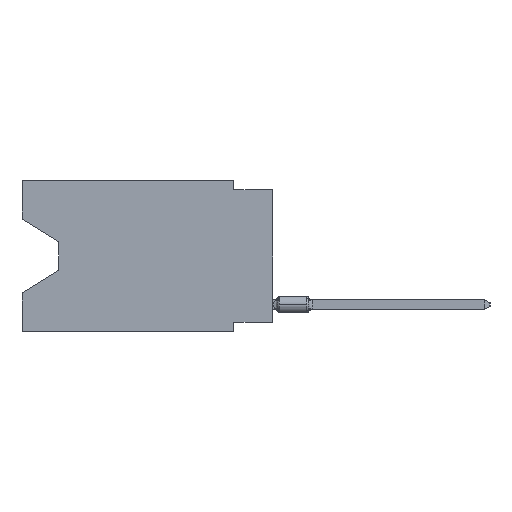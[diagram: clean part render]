
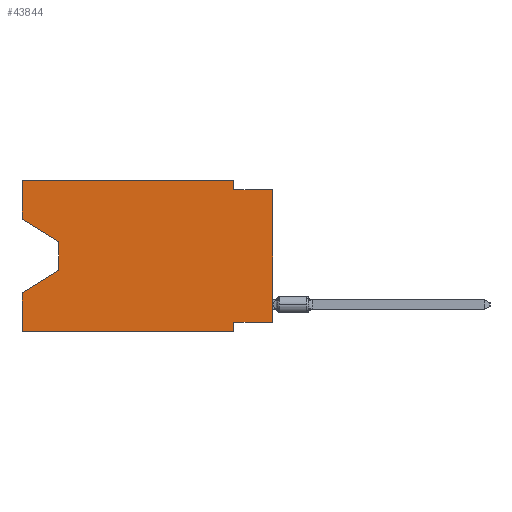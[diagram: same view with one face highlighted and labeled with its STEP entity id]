
A CAD part, left-side view. The second image highlights one B-rep face of the part: STEP entity #43844.
In plain terms, the highlighted planar face has unit normal (-1, 0, 0).
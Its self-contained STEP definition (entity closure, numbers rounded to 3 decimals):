
#414 = LINE ( 'NONE', #41570, #20979 ) ;
#594 = LINE ( 'NONE', #4334, #33342 ) ;
#1534 = DIRECTION ( 'NONE',  ( 0., 0., -1. ) ) ;
#2400 = ORIENTED_EDGE ( 'NONE', *, *, #45570, .F. ) ;
#2598 = DIRECTION ( 'NONE',  ( 1., 0., 0. ) ) ;
#3340 = CARTESIAN_POINT ( 'NONE',  ( 0., 2.54, -9.906 ) ) ;
#4219 = EDGE_CURVE ( 'NONE', #40050, #27519, #4871, .T. ) ;
#4334 = CARTESIAN_POINT ( 'NONE',  ( 0., 13.97, -5.893 ) ) ;
#4600 = DIRECTION ( 'NONE',  ( 0., 1., 0. ) ) ;
#4824 = LINE ( 'NONE', #29526, #19362 ) ;
#4871 = LINE ( 'NONE', #29850, #43317 ) ;
#5742 = CARTESIAN_POINT ( 'NONE',  ( 0., 2.54, 0. ) ) ;
#6834 = AXIS2_PLACEMENT_3D ( 'NONE', #39268, #2598, #22293 ) ;
#7279 = VECTOR ( 'NONE', #7648, 1000. ) ;
#7379 = LINE ( 'NONE', #43779, #7279 ) ;
#7648 = DIRECTION ( 'NONE',  ( 0., 0., 1. ) ) ;
#7811 = CARTESIAN_POINT ( 'NONE',  ( 0., 16.383, -7.36 ) ) ;
#8549 = DIRECTION ( 'NONE',  ( 0., -1., 0. ) ) ;
#8772 = ORIENTED_EDGE ( 'NONE', *, *, #42619, .F. ) ;
#8884 = EDGE_CURVE ( 'NONE', #28193, #33493, #33404, .T. ) ;
#9623 = LINE ( 'NONE', #21852, #44292 ) ;
#9801 = VERTEX_POINT ( 'NONE', #40774 ) ;
#9888 = EDGE_CURVE ( 'NONE', #28742, #27519, #44262, .T. ) ;
#12550 = LINE ( 'NONE', #24804, #28298 ) ;
#12706 = CARTESIAN_POINT ( 'NONE',  ( 0., 2.54, -9.906 ) ) ;
#13138 = CARTESIAN_POINT ( 'NONE',  ( 0., 2.54, -0.635 ) ) ;
#13321 = ORIENTED_EDGE ( 'NONE', *, *, #9888, .F. ) ;
#15783 = CARTESIAN_POINT ( 'NONE',  ( 0., 16.383, -2.546 ) ) ;
#15956 = VERTEX_POINT ( 'NONE', #13138 ) ;
#16697 = CARTESIAN_POINT ( 'NONE',  ( 0., 16.383, 0. ) ) ;
#19323 = CARTESIAN_POINT ( 'NONE',  ( 0., 16.383, -9.906 ) ) ;
#19362 = VECTOR ( 'NONE', #8549, 1000. ) ;
#19572 = DIRECTION ( 'NONE',  ( 0., 0., -1. ) ) ;
#20979 = VECTOR ( 'NONE', #41314, 1000. ) ;
#21483 = VERTEX_POINT ( 'NONE', #49431 ) ;
#21852 = CARTESIAN_POINT ( 'NONE',  ( 0., 16.383, 0. ) ) ;
#22277 = LINE ( 'NONE', #26261, #51580 ) ;
#22293 = DIRECTION ( 'NONE',  ( 0., 0., -1. ) ) ;
#22459 = LINE ( 'NONE', #47402, #42807 ) ;
#23095 = FACE_OUTER_BOUND ( 'NONE', #48795, .T. ) ;
#23185 = EDGE_CURVE ( 'NONE', #33493, #15956, #22277, .T. ) ;
#24553 = VECTOR ( 'NONE', #27745, 1000. ) ;
#24804 = CARTESIAN_POINT ( 'NONE',  ( 0., 0., -9.271 ) ) ;
#26261 = CARTESIAN_POINT ( 'NONE',  ( 0., 2.54, 0. ) ) ;
#26876 = EDGE_CURVE ( 'NONE', #30911, #21483, #22459, .T. ) ;
#27298 = ORIENTED_EDGE ( 'NONE', *, *, #35613, .F. ) ;
#27519 = VERTEX_POINT ( 'NONE', #12706 ) ;
#27745 = DIRECTION ( 'NONE',  ( 0., -0.855, -0.519 ) ) ;
#28193 = VERTEX_POINT ( 'NONE', #47946 ) ;
#28298 = VECTOR ( 'NONE', #4600, 1000. ) ;
#28742 = VERTEX_POINT ( 'NONE', #30296 ) ;
#28753 = ORIENTED_EDGE ( 'NONE', *, *, #48806, .T. ) ;
#29526 = CARTESIAN_POINT ( 'NONE',  ( 0., 0., -0.635 ) ) ;
#29850 = CARTESIAN_POINT ( 'NONE',  ( 0., 16.383, -9.906 ) ) ;
#30296 = CARTESIAN_POINT ( 'NONE',  ( 0., 2.54, -9.271 ) ) ;
#30537 = ORIENTED_EDGE ( 'NONE', *, *, #50709, .F. ) ;
#30911 = VERTEX_POINT ( 'NONE', #33402 ) ;
#31215 = DIRECTION ( 'NONE',  ( 0., 0., -1. ) ) ;
#32739 = VERTEX_POINT ( 'NONE', #7811 ) ;
#32745 = VERTEX_POINT ( 'NONE', #43329 ) ;
#32897 = DIRECTION ( 'NONE',  ( 0., -1., 0. ) ) ;
#33342 = VECTOR ( 'NONE', #44715, 1000. ) ;
#33402 = CARTESIAN_POINT ( 'NONE',  ( 0., 13.97, -4.013 ) ) ;
#33404 = LINE ( 'NONE', #16697, #41034 ) ;
#33493 = VERTEX_POINT ( 'NONE', #5742 ) ;
#34555 = ORIENTED_EDGE ( 'NONE', *, *, #52411, .T. ) ;
#35613 = EDGE_CURVE ( 'NONE', #35657, #28193, #9623, .T. ) ;
#35657 = VERTEX_POINT ( 'NONE', #43868 ) ;
#36634 = ORIENTED_EDGE ( 'NONE', *, *, #26876, .T. ) ;
#38558 = DIRECTION ( 'NONE',  ( 0., 0., 1. ) ) ;
#38993 = PLANE ( 'NONE',  #6834 ) ;
#39173 = ORIENTED_EDGE ( 'NONE', *, *, #45615, .T. ) ;
#39268 = CARTESIAN_POINT ( 'NONE',  ( 0., 16.383, 0. ) ) ;
#40050 = VERTEX_POINT ( 'NONE', #19323 ) ;
#40774 = CARTESIAN_POINT ( 'NONE',  ( 0., 0., -9.271 ) ) ;
#41034 = VECTOR ( 'NONE', #32897, 1000. ) ;
#41213 = ORIENTED_EDGE ( 'NONE', *, *, #4219, .T. ) ;
#41314 = DIRECTION ( 'NONE',  ( 0., 0., 1. ) ) ;
#41517 = DIRECTION ( 'NONE',  ( 0., -1., 0. ) ) ;
#41570 = CARTESIAN_POINT ( 'NONE',  ( 0., 0., 0. ) ) ;
#42112 = ORIENTED_EDGE ( 'NONE', *, *, #8884, .F. ) ;
#42619 = EDGE_CURVE ( 'NONE', #40050, #32739, #7379, .T. ) ;
#42807 = VECTOR ( 'NONE', #31215, 1000. ) ;
#43317 = VECTOR ( 'NONE', #41517, 1000. ) ;
#43329 = CARTESIAN_POINT ( 'NONE',  ( 0., 0., -0.635 ) ) ;
#43779 = CARTESIAN_POINT ( 'NONE',  ( 0., 16.383, 0. ) ) ;
#43844 = ADVANCED_FACE ( 'NONE', ( #23095 ), #38993, .F. ) ;
#43868 = CARTESIAN_POINT ( 'NONE',  ( 0., 16.383, -2.546 ) ) ;
#44262 = LINE ( 'NONE', #3340, #45366 ) ;
#44292 = VECTOR ( 'NONE', #38558, 1000. ) ;
#44715 = DIRECTION ( 'NONE',  ( 0., 0.855, -0.519 ) ) ;
#45366 = VECTOR ( 'NONE', #19572, 1000. ) ;
#45570 = EDGE_CURVE ( 'NONE', #9801, #28742, #12550, .T. ) ;
#45615 = EDGE_CURVE ( 'NONE', #21483, #32739, #594, .T. ) ;
#47402 = CARTESIAN_POINT ( 'NONE',  ( 0., 13.97, -4.013 ) ) ;
#47946 = CARTESIAN_POINT ( 'NONE',  ( 0., 16.383, 0. ) ) ;
#48430 = LINE ( 'NONE', #15783, #24553 ) ;
#48795 = EDGE_LOOP ( 'NONE', ( #34555, #36634, #39173, #8772, #41213, #13321, #2400, #28753, #30537, #50942, #42112, #27298 ) ) ;
#48806 = EDGE_CURVE ( 'NONE', #9801, #32745, #414, .T. ) ;
#49431 = CARTESIAN_POINT ( 'NONE',  ( 0., 13.97, -5.893 ) ) ;
#50709 = EDGE_CURVE ( 'NONE', #15956, #32745, #4824, .T. ) ;
#50942 = ORIENTED_EDGE ( 'NONE', *, *, #23185, .F. ) ;
#51580 = VECTOR ( 'NONE', #1534, 1000. ) ;
#52411 = EDGE_CURVE ( 'NONE', #35657, #30911, #48430, .T. ) ;
